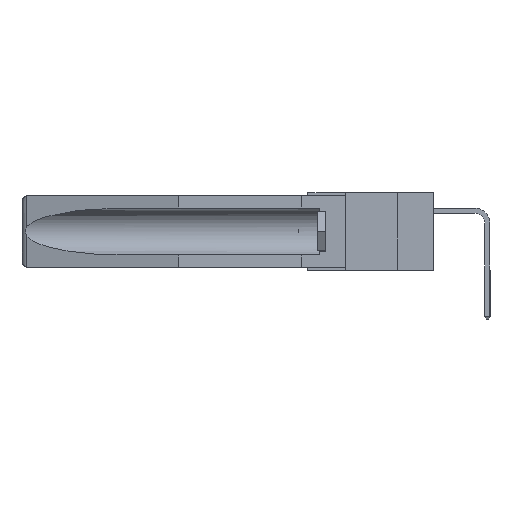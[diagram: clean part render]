
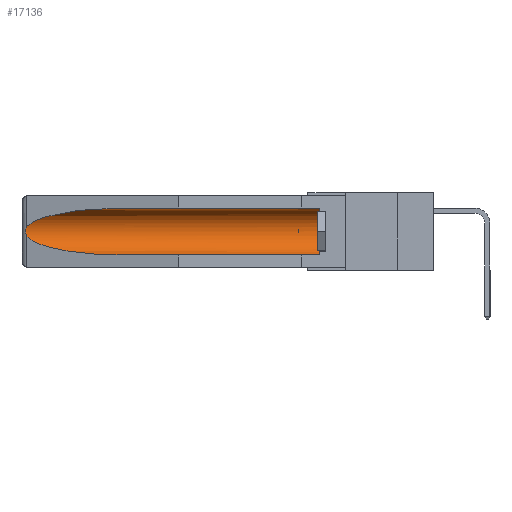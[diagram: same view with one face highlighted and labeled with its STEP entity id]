
A CAD part, left-side view. The second image highlights one B-rep face of the part: STEP entity #17136.
In plain terms, the highlighted cylindrical face has radius 2.857 mm (diameter 5.715 mm), a partial arc.
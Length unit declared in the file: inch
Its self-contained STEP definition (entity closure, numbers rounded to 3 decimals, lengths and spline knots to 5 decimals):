
#94 = DIRECTION ( 'NONE',  ( 0., 1., 0. ) ) ;
#373 = CARTESIAN_POINT ( 'NONE',  ( 0.2673, 1.5327, -0.16383 ) ) ;
#702 = VERTEX_POINT ( 'NONE', #11022 ) ;
#831 = CARTESIAN_POINT ( 'NONE',  ( 0.26597, 1.5296, -0.19026 ) ) ;
#2163 = LINE ( 'NONE', #3498, #21364 ) ;
#2570 = CARTESIAN_POINT ( 'NONE',  ( 0.155, 0.126, -0.1715 ) ) ;
#3041 = CARTESIAN_POINT ( 'NONE',  ( 0.2673, 1.53269, -0.17917 ) ) ;
#3498 = CARTESIAN_POINT ( 'NONE',  ( 0.155, -0.30754, -0.284 ) ) ;
#5554 = CARTESIAN_POINT ( 'NONE',  ( 0.25451, 1.48313, -0.09465 ) ) ;
#7665 = CYLINDRICAL_SURFACE ( 'NONE', #9855, 0.1125 ) ;
#8534 = CARTESIAN_POINT ( 'NONE',  ( 0.2675, 1.53308, -0.17534 ) ) ;
#8540 = EDGE_CURVE ( 'NONE', #702, #32748, #2163, .T. ) ;
#8895 = ORIENTED_EDGE ( 'NONE', *, *, #25928, .T. ) ;
#9855 = AXIS2_PLACEMENT_3D ( 'NONE', #24917, #24686, #33176 ) ;
#10249 = EDGE_CURVE ( 'NONE', #33128, #27619, #11564, .T. ) ;
#10709 = CARTESIAN_POINT ( 'NONE',  ( 0.21114, 1.30732, -0.059 ) ) ;
#11022 = CARTESIAN_POINT ( 'NONE',  ( 0.155, 0.126, -0.284 ) ) ;
#11564 = B_SPLINE_CURVE_WITH_KNOTS ( 'NONE', 3,
 ( #27308, #32874, #19482, #373, #30209, #8534, #3041, #21710, #831, #16690 ),
 .UNSPECIFIED., .F., .F.,
 ( 4, 2, 2, 2, 4 ),
 ( 0., 0.00029, 0.00058, 0.00087, 0.00117 ),
 .UNSPECIFIED. ) ;
#11891 = ORIENTED_EDGE ( 'NONE', *, *, #8540, .F. ) ;
#13268 = CARTESIAN_POINT ( 'NONE',  ( 0.21114, 1.30732, -0.284 ) ) ;
#13820 = CARTESIAN_POINT ( 'NONE',  ( 0.155, -0.30754, -0.059 ) ) ;
#14383 = CARTESIAN_POINT ( 'NONE',  ( 0.26537, 1.52718, -0.14972 ) ) ;
#16199 = CARTESIAN_POINT ( 'NONE',  ( 0.155, 1.07973, -0.284 ) ) ;
#16647 = LINE ( 'NONE', #13820, #28322 ) ;
#16690 = CARTESIAN_POINT ( 'NONE',  ( 0.26537, 1.52718, -0.19328 ) ) ;
#17136 = ADVANCED_FACE ( 'NONE', ( #24758 ), #7665, .F. ) ;
#18384 =( BOUNDED_CURVE ( )  B_SPLINE_CURVE ( 3, ( #24083, #29688, #13268, #16199 ),
 .UNSPECIFIED., .F., .F. ) 
 B_SPLINE_CURVE_WITH_KNOTS ( ( 4, 4 ),
 ( 0.1948, 1.5708 ),
 .UNSPECIFIED. ) 
 CURVE ( )  GEOMETRIC_REPRESENTATION_ITEM ( )  RATIONAL_B_SPLINE_CURVE ( ( 1., 0.848, 0.848, 1. ) ) 
 REPRESENTATION_ITEM ( '' )  );
#18690 = AXIS2_PLACEMENT_3D ( 'NONE', #2570, #21597, #31723 ) ;
#18978 = VERTEX_POINT ( 'NONE', #20708 ) ;
#19277 = ORIENTED_EDGE ( 'NONE', *, *, #10249, .T. ) ;
#19482 = CARTESIAN_POINT ( 'NONE',  ( 0.26654, 1.53092, -0.15636 ) ) ;
#20708 = CARTESIAN_POINT ( 'NONE',  ( 0.155, 1.07973, -0.059 ) ) ;
#20823 = CARTESIAN_POINT ( 'NONE',  ( 0.155, 1.07973, -0.284 ) ) ;
#20912 = VERTEX_POINT ( 'NONE', #34480 ) ;
#21340 = CARTESIAN_POINT ( 'NONE',  ( 0.155, 1.07973, -0.059 ) ) ;
#21364 = VECTOR ( 'NONE', #27769, 39.37008 ) ;
#21597 = DIRECTION ( 'NONE',  ( 0., -1., 0. ) ) ;
#21710 = CARTESIAN_POINT ( 'NONE',  ( 0.26655, 1.53094, -0.18657 ) ) ;
#21976 = ORIENTED_EDGE ( 'NONE', *, *, #26306, .T. ) ;
#22032 = CARTESIAN_POINT ( 'NONE',  ( 0.26537, 1.52718, -0.19328 ) ) ;
#22292 = ORIENTED_EDGE ( 'NONE', *, *, #23540, .T. ) ;
#23461 = CIRCLE ( 'NONE', #18690, 0.1125 ) ;
#23540 = EDGE_CURVE ( 'NONE', #18978, #33128, #33772, .T. ) ;
#23913 = EDGE_CURVE ( 'NONE', #20912, #18978, #16647, .T. ) ;
#24083 = CARTESIAN_POINT ( 'NONE',  ( 0.26537, 1.52718, -0.19328 ) ) ;
#24215 = CARTESIAN_POINT ( 'NONE',  ( 0.26537, 1.52718, -0.14972 ) ) ;
#24686 = DIRECTION ( 'NONE',  ( 0., 1., 0. ) ) ;
#24758 = FACE_OUTER_BOUND ( 'NONE', #28764, .T. ) ;
#24917 = CARTESIAN_POINT ( 'NONE',  ( 0.155, -0.30754, -0.1715 ) ) ;
#25928 = EDGE_CURVE ( 'NONE', #702, #20912, #23461, .T. ) ;
#26306 = EDGE_CURVE ( 'NONE', #27619, #32748, #18384, .T. ) ;
#27308 = CARTESIAN_POINT ( 'NONE',  ( 0.26537, 1.52718, -0.14972 ) ) ;
#27619 = VERTEX_POINT ( 'NONE', #22032 ) ;
#27769 = DIRECTION ( 'NONE',  ( 0., 1., 0. ) ) ;
#28322 = VECTOR ( 'NONE', #94, 39.37008 ) ;
#28764 = EDGE_LOOP ( 'NONE', ( #22292, #19277, #21976, #11891, #8895, #32095 ) ) ;
#29688 = CARTESIAN_POINT ( 'NONE',  ( 0.25451, 1.48313, -0.24835 ) ) ;
#30209 = CARTESIAN_POINT ( 'NONE',  ( 0.2675, 1.53308, -0.16763 ) ) ;
#31723 = DIRECTION ( 'NONE',  ( 0., 0., 1. ) ) ;
#32095 = ORIENTED_EDGE ( 'NONE', *, *, #23913, .T. ) ;
#32748 = VERTEX_POINT ( 'NONE', #20823 ) ;
#32874 = CARTESIAN_POINT ( 'NONE',  ( 0.26597, 1.52961, -0.15275 ) ) ;
#33128 = VERTEX_POINT ( 'NONE', #14383 ) ;
#33176 = DIRECTION ( 'NONE',  ( 0., 0., 1. ) ) ;
#33772 =( BOUNDED_CURVE ( )  B_SPLINE_CURVE ( 3, ( #21340, #10709, #5554, #24215 ),
 .UNSPECIFIED., .F., .F. ) 
 B_SPLINE_CURVE_WITH_KNOTS ( ( 4, 4 ),
 ( 4.71239, 6.08839 ),
 .UNSPECIFIED. ) 
 CURVE ( )  GEOMETRIC_REPRESENTATION_ITEM ( )  RATIONAL_B_SPLINE_CURVE ( ( 1., 0.848, 0.848, 1. ) ) 
 REPRESENTATION_ITEM ( '' )  );
#34480 = CARTESIAN_POINT ( 'NONE',  ( 0.155, 0.126, -0.059 ) ) ;
